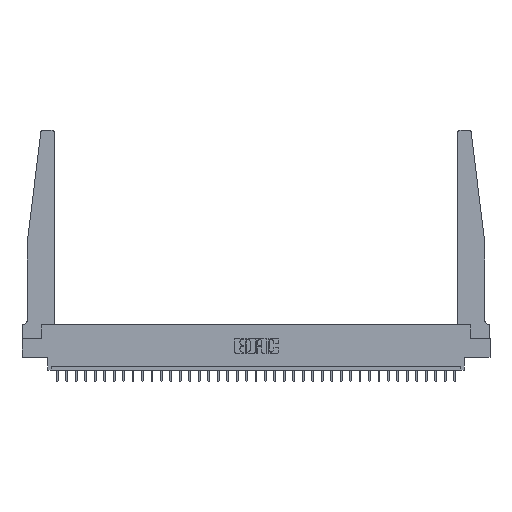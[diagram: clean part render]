
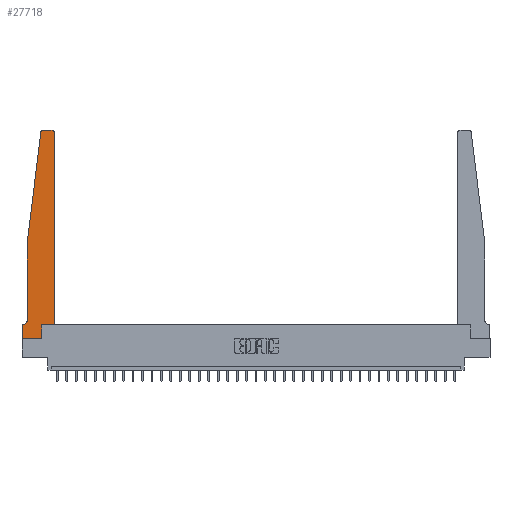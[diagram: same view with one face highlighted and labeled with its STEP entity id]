
A CAD part, top view. The second image highlights one B-rep face of the part: STEP entity #27718.
In plain terms, the highlighted planar face has unit normal (0, 0, 1).
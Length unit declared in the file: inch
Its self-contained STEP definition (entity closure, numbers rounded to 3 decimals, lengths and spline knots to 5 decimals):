
#293 = CARTESIAN_POINT ( 'NONE',  ( 0.065, 0.1875, 0.37 ) ) ;
#706 = VERTEX_POINT ( 'NONE', #28669 ) ;
#780 = VECTOR ( 'NONE', #18863, 39.37008 ) ;
#1074 = CARTESIAN_POINT ( 'NONE',  ( 0., 0.1875, 0.37 ) ) ;
#1291 = AXIS2_PLACEMENT_3D ( 'NONE', #8532, #10661, #25503 ) ;
#1540 = ORIENTED_EDGE ( 'NONE', *, *, #17247, .T. ) ;
#1586 = VERTEX_POINT ( 'NONE', #1074 ) ;
#1647 = DIRECTION ( 'NONE',  ( 1., 0., 0. ) ) ;
#1832 = EDGE_CURVE ( 'NONE', #14545, #4725, #14978, .T. ) ;
#2263 = VERTEX_POINT ( 'NONE', #7688 ) ;
#2754 = DIRECTION ( 'NONE',  ( 1., 0., 0. ) ) ;
#2860 = CARTESIAN_POINT ( 'NONE',  ( 0.2605, 0.18, 0.37 ) ) ;
#2950 = CARTESIAN_POINT ( 'NONE',  ( 0.425, 0.18, 0.37 ) ) ;
#3066 = DIRECTION ( 'NONE',  ( 0., 1., 0. ) ) ;
#3237 = VECTOR ( 'NONE', #1647, 39.37008 ) ;
#3907 = AXIS2_PLACEMENT_3D ( 'NONE', #7126, #11600, #16818 ) ;
#4044 = LINE ( 'NONE', #30378, #16198 ) ;
#4556 = CIRCLE ( 'NONE', #17347, 0.03 ) ;
#4725 = VERTEX_POINT ( 'NONE', #13658 ) ;
#5185 = EDGE_CURVE ( 'NONE', #20815, #8372, #4556, .T. ) ;
#6865 = CARTESIAN_POINT ( 'NONE',  ( 0.27653, 2.72, 0.37 ) ) ;
#7126 = CARTESIAN_POINT ( 'NONE',  ( 0.015, 0.2375, 0.37 ) ) ;
#7299 = VECTOR ( 'NONE', #22301, 39.37008 ) ;
#7363 = CARTESIAN_POINT ( 'NONE',  ( 0.425, 2.72, 0.37 ) ) ;
#7688 = CARTESIAN_POINT ( 'NONE',  ( 0.2605, 0., 0.37 ) ) ;
#8184 = DIRECTION ( 'NONE',  ( -0.122, -0.992, 0. ) ) ;
#8372 = VERTEX_POINT ( 'NONE', #29752 ) ;
#8532 = CARTESIAN_POINT ( 'NONE',  ( 0., 0.1875, 0.37 ) ) ;
#8535 = VECTOR ( 'NONE', #27077, 39.37008 ) ;
#8552 = EDGE_CURVE ( 'NONE', #29039, #9373, #15332, .T. ) ;
#9373 = VERTEX_POINT ( 'NONE', #7363 ) ;
#9430 = LINE ( 'NONE', #27484, #10193 ) ;
#9561 = CARTESIAN_POINT ( 'NONE',  ( 0.395, 2.72, 0.37 ) ) ;
#9764 = LINE ( 'NONE', #30517, #27573 ) ;
#10162 = ORIENTED_EDGE ( 'NONE', *, *, #22326, .T. ) ;
#10193 = VECTOR ( 'NONE', #8184, 39.37008 ) ;
#10477 = ORIENTED_EDGE ( 'NONE', *, *, #26325, .T. ) ;
#10661 = DIRECTION ( 'NONE',  ( 0., 0., 1. ) ) ;
#10879 = CARTESIAN_POINT ( 'NONE',  ( 0.425, 0.18, 0.37 ) ) ;
#11290 = EDGE_CURVE ( 'NONE', #8372, #14545, #9430, .T. ) ;
#11600 = DIRECTION ( 'NONE',  ( 0., 0., -1. ) ) ;
#11761 = VERTEX_POINT ( 'NONE', #15507 ) ;
#11888 = ORIENTED_EDGE ( 'NONE', *, *, #28289, .T. ) ;
#12089 = CIRCLE ( 'NONE', #3907, 0.05 ) ;
#12506 = CARTESIAN_POINT ( 'NONE',  ( 0.425, 0.18, 0.37 ) ) ;
#12529 = AXIS2_PLACEMENT_3D ( 'NONE', #9561, #24314, #2754 ) ;
#12997 = CIRCLE ( 'NONE', #12529, 0.03 ) ;
#13658 = CARTESIAN_POINT ( 'NONE',  ( 0.065, 0.2375, 0.37 ) ) ;
#14271 = CARTESIAN_POINT ( 'NONE',  ( 0., 0., 0.37 ) ) ;
#14288 = LINE ( 'NONE', #12506, #26454 ) ;
#14545 = VERTEX_POINT ( 'NONE', #29656 ) ;
#14978 = LINE ( 'NONE', #24858, #8535 ) ;
#15332 = LINE ( 'NONE', #2950, #27474 ) ;
#15507 = CARTESIAN_POINT ( 'NONE',  ( 0.015, 0.1875, 0.37 ) ) ;
#15628 = EDGE_CURVE ( 'NONE', #11761, #1586, #16352, .T. ) ;
#15968 = ORIENTED_EDGE ( 'NONE', *, *, #1832, .T. ) ;
#16074 = DIRECTION ( 'NONE',  ( -1., 0., 0. ) ) ;
#16198 = VECTOR ( 'NONE', #18028, 39.37008 ) ;
#16352 = LINE ( 'NONE', #293, #780 ) ;
#16818 = DIRECTION ( 'NONE',  ( -1., 0., 0. ) ) ;
#16897 = LINE ( 'NONE', #14271, #3237 ) ;
#17247 = EDGE_CURVE ( 'NONE', #23881, #20815, #9764, .T. ) ;
#17347 = AXIS2_PLACEMENT_3D ( 'NONE', #6865, #28954, #31117 ) ;
#17512 = ORIENTED_EDGE ( 'NONE', *, *, #5185, .T. ) ;
#18028 = DIRECTION ( 'NONE',  ( 0., -1., 0. ) ) ;
#18308 = ORIENTED_EDGE ( 'NONE', *, *, #8552, .T. ) ;
#18863 = DIRECTION ( 'NONE',  ( -1., 0., 0. ) ) ;
#19383 = ORIENTED_EDGE ( 'NONE', *, *, #27357, .T. ) ;
#19469 = CARTESIAN_POINT ( 'NONE',  ( 0.2605, 0.18, 0.37 ) ) ;
#19997 = ORIENTED_EDGE ( 'NONE', *, *, #25447, .T. ) ;
#20084 = EDGE_CURVE ( 'NONE', #9373, #23881, #12997, .T. ) ;
#20812 = ORIENTED_EDGE ( 'NONE', *, *, #11290, .T. ) ;
#20815 = VERTEX_POINT ( 'NONE', #23474 ) ;
#21406 = CARTESIAN_POINT ( 'NONE',  ( 0.395, 2.75, 0.37 ) ) ;
#22301 = DIRECTION ( 'NONE',  ( 0., 1., 0. ) ) ;
#22326 = EDGE_CURVE ( 'NONE', #2263, #28144, #26674, .T. ) ;
#22500 = DIRECTION ( 'NONE',  ( 1., 0., 0. ) ) ;
#23297 = ORIENTED_EDGE ( 'NONE', *, *, #20084, .T. ) ;
#23474 = CARTESIAN_POINT ( 'NONE',  ( 0.27653, 2.75, 0.37 ) ) ;
#23881 = VERTEX_POINT ( 'NONE', #21406 ) ;
#24314 = DIRECTION ( 'NONE',  ( 0., 0., 1. ) ) ;
#24858 = CARTESIAN_POINT ( 'NONE',  ( 0.065, 1.25, 0.37 ) ) ;
#25318 = FACE_OUTER_BOUND ( 'NONE', #28661, .T. ) ;
#25447 = EDGE_CURVE ( 'NONE', #4725, #11761, #12089, .T. ) ;
#25503 = DIRECTION ( 'NONE',  ( 1., 0., 0. ) ) ;
#25864 = ORIENTED_EDGE ( 'NONE', *, *, #15628, .T. ) ;
#26325 = EDGE_CURVE ( 'NONE', #28144, #29039, #14288, .T. ) ;
#26454 = VECTOR ( 'NONE', #22500, 39.37008 ) ;
#26674 = LINE ( 'NONE', #2860, #7299 ) ;
#27077 = DIRECTION ( 'NONE',  ( 0., -1., 0. ) ) ;
#27357 = EDGE_CURVE ( 'NONE', #706, #2263, #16897, .T. ) ;
#27474 = VECTOR ( 'NONE', #3066, 39.37008 ) ;
#27484 = CARTESIAN_POINT ( 'NONE',  ( 0.065, 1.25, 0.37 ) ) ;
#27573 = VECTOR ( 'NONE', #16074, 39.37008 ) ;
#27599 = PLANE ( 'NONE',  #1291 ) ;
#27718 = ADVANCED_FACE ( 'NONE', ( #25318 ), #27599, .T. ) ;
#28144 = VERTEX_POINT ( 'NONE', #19469 ) ;
#28289 = EDGE_CURVE ( 'NONE', #1586, #706, #4044, .T. ) ;
#28661 = EDGE_LOOP ( 'NONE', ( #1540, #17512, #20812, #15968, #19997, #25864, #11888, #19383, #10162, #10477, #18308, #23297 ) ) ;
#28669 = CARTESIAN_POINT ( 'NONE',  ( 0., 0., 0.37 ) ) ;
#28954 = DIRECTION ( 'NONE',  ( 0., 0., 1. ) ) ;
#29039 = VERTEX_POINT ( 'NONE', #10879 ) ;
#29656 = CARTESIAN_POINT ( 'NONE',  ( 0.065, 1.25, 0.37 ) ) ;
#29752 = CARTESIAN_POINT ( 'NONE',  ( 0.24675, 2.72367, 0.37 ) ) ;
#30378 = CARTESIAN_POINT ( 'NONE',  ( 0., 0., 0.37 ) ) ;
#30517 = CARTESIAN_POINT ( 'NONE',  ( 0.25, 2.75, 0.37 ) ) ;
#31117 = DIRECTION ( 'NONE',  ( 1., 0., 0. ) ) ;
